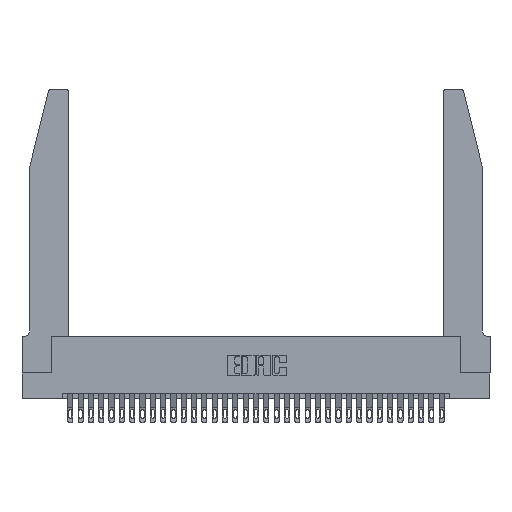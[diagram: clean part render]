
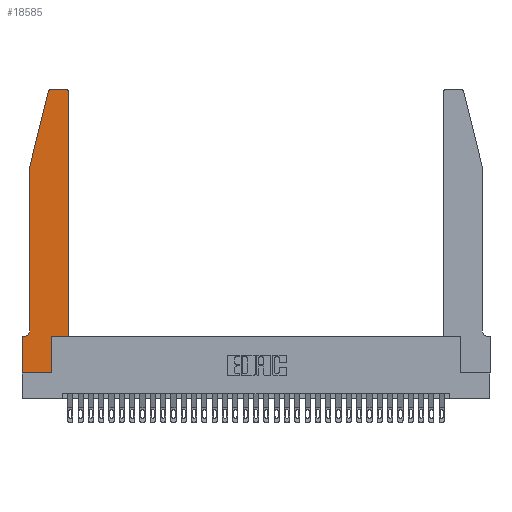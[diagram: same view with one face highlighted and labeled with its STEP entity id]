
A CAD part, top view. The second image highlights one B-rep face of the part: STEP entity #18585.
In plain terms, the highlighted planar face has unit normal (0, 0, 1).
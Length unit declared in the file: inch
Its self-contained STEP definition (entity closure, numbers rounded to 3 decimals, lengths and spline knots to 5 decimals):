
#20 = EDGE_LOOP ( 'NONE', ( #24383, #28133, #33479, #28263, #9314, #33963, #3796, #21470, #34028, #24798, #11192, #2394 ) ) ;
#1036 = DIRECTION ( 'NONE',  ( 0., 1., 0. ) ) ;
#1741 = DIRECTION ( 'NONE',  ( 1., 0., 0. ) ) ;
#1934 = AXIS2_PLACEMENT_3D ( 'NONE', #31830, #33931, #18137 ) ;
#2394 = ORIENTED_EDGE ( 'NONE', *, *, #11421, .T. ) ;
#2669 = VECTOR ( 'NONE', #12500, 39.37008 ) ;
#3556 = EDGE_CURVE ( 'NONE', #12029, #30314, #17041, .T. ) ;
#3796 = ORIENTED_EDGE ( 'NONE', *, *, #12665, .T. ) ;
#3810 = LINE ( 'NONE', #32622, #26103 ) ;
#4499 = LINE ( 'NONE', #11908, #25490 ) ;
#4633 = LINE ( 'NONE', #25714, #8369 ) ;
#5110 = VERTEX_POINT ( 'NONE', #10201 ) ;
#5418 = VERTEX_POINT ( 'NONE', #31529 ) ;
#5482 = VERTEX_POINT ( 'NONE', #34102 ) ;
#5614 = EDGE_CURVE ( 'NONE', #20207, #5418, #29988, .T. ) ;
#6049 = DIRECTION ( 'NONE',  ( 1., 0., 0. ) ) ;
#6321 = CARTESIAN_POINT ( 'NONE',  ( 0.4505, 2.72, 0.37 ) ) ;
#6489 = EDGE_CURVE ( 'NONE', #10993, #6961, #17718, .T. ) ;
#6961 = VERTEX_POINT ( 'NONE', #12233 ) ;
#7520 = VECTOR ( 'NONE', #23415, 39.37008 ) ;
#8369 = VECTOR ( 'NONE', #31286, 39.37008 ) ;
#8616 = CARTESIAN_POINT ( 'NONE',  ( 0., 0.35, 0.37 ) ) ;
#9282 = EDGE_CURVE ( 'NONE', #5418, #12029, #10143, .T. ) ;
#9314 = ORIENTED_EDGE ( 'NONE', *, *, #3556, .T. ) ;
#9832 = EDGE_CURVE ( 'NONE', #5110, #13591, #3810, .T. ) ;
#10000 = VERTEX_POINT ( 'NONE', #6321 ) ;
#10143 = LINE ( 'NONE', #28679, #30764 ) ;
#10201 = CARTESIAN_POINT ( 'NONE',  ( 0.4205, 2.75, 0.37 ) ) ;
#10918 = CARTESIAN_POINT ( 'NONE',  ( 0.25487, 2.72718, 0.37 ) ) ;
#10931 = EDGE_CURVE ( 'NONE', #27137, #5482, #4633, .T. ) ;
#10993 = VERTEX_POINT ( 'NONE', #21674 ) ;
#11192 = ORIENTED_EDGE ( 'NONE', *, *, #14235, .T. ) ;
#11421 = EDGE_CURVE ( 'NONE', #10000, #5110, #16294, .T. ) ;
#11894 = AXIS2_PLACEMENT_3D ( 'NONE', #8616, #19373, #6049 ) ;
#11908 = CARTESIAN_POINT ( 'NONE',  ( 0., 0., 0.37 ) ) ;
#12029 = VERTEX_POINT ( 'NONE', #34087 ) ;
#12233 = CARTESIAN_POINT ( 'NONE',  ( 0.4505, 0.35, 0.37 ) ) ;
#12500 = DIRECTION ( 'NONE',  ( -0.239, -0.971, 0. ) ) ;
#12665 = EDGE_CURVE ( 'NONE', #13957, #27137, #4499, .T. ) ;
#12746 = CIRCLE ( 'NONE', #1934, 0.03 ) ;
#13058 = CARTESIAN_POINT ( 'NONE',  ( 0., 0.35, 0.37 ) ) ;
#13591 = VERTEX_POINT ( 'NONE', #25561 ) ;
#13957 = VERTEX_POINT ( 'NONE', #13058 ) ;
#14192 = CARTESIAN_POINT ( 'NONE',  ( 0.4505, 0.35, 0.37 ) ) ;
#14235 = EDGE_CURVE ( 'NONE', #6961, #10000, #25348, .T. ) ;
#15864 = LINE ( 'NONE', #33928, #7520 ) ;
#16294 = CIRCLE ( 'NONE', #24153, 0.03 ) ;
#16435 = LINE ( 'NONE', #25525, #33722 ) ;
#17041 = CIRCLE ( 'NONE', #17306, 0.07 ) ;
#17306 = AXIS2_PLACEMENT_3D ( 'NONE', #25915, #20619, #22845 ) ;
#17718 = LINE ( 'NONE', #19577, #33281 ) ;
#18137 = DIRECTION ( 'NONE',  ( 1., 0., 0. ) ) ;
#18141 = EDGE_CURVE ( 'NONE', #30314, #13957, #16435, .T. ) ;
#18178 = DIRECTION ( 'NONE',  ( 0., 0., 1. ) ) ;
#18585 = ADVANCED_FACE ( 'NONE', ( #23561 ), #21867, .T. ) ;
#19373 = DIRECTION ( 'NONE',  ( 0., 0., 1. ) ) ;
#19577 = CARTESIAN_POINT ( 'NONE',  ( 0.4505, 0.35, 0.37 ) ) ;
#20207 = VERTEX_POINT ( 'NONE', #10918 ) ;
#20246 = DIRECTION ( 'NONE',  ( 0., -1., 0. ) ) ;
#20619 = DIRECTION ( 'NONE',  ( 0., 0., -1. ) ) ;
#20823 = CARTESIAN_POINT ( 'NONE',  ( 0.0755, 2., 0.37 ) ) ;
#21470 = ORIENTED_EDGE ( 'NONE', *, *, #10931, .T. ) ;
#21674 = CARTESIAN_POINT ( 'NONE',  ( 0.2865, 0.35, 0.37 ) ) ;
#21867 = PLANE ( 'NONE',  #11894 ) ;
#22329 = DIRECTION ( 'NONE',  ( -1., 0., 0. ) ) ;
#22604 = EDGE_CURVE ( 'NONE', #13591, #20207, #12746, .T. ) ;
#22845 = DIRECTION ( 'NONE',  ( -1., 0., 0. ) ) ;
#23415 = DIRECTION ( 'NONE',  ( 0., 1., 0. ) ) ;
#23561 = FACE_OUTER_BOUND ( 'NONE', #20, .T. ) ;
#24153 = AXIS2_PLACEMENT_3D ( 'NONE', #34327, #18178, #31867 ) ;
#24383 = ORIENTED_EDGE ( 'NONE', *, *, #9832, .T. ) ;
#24798 = ORIENTED_EDGE ( 'NONE', *, *, #6489, .T. ) ;
#25348 = LINE ( 'NONE', #14192, #32127 ) ;
#25490 = VECTOR ( 'NONE', #20246, 39.37008 ) ;
#25525 = CARTESIAN_POINT ( 'NONE',  ( 0.0755, 0.35, 0.37 ) ) ;
#25561 = CARTESIAN_POINT ( 'NONE',  ( 0.284, 2.75, 0.37 ) ) ;
#25714 = CARTESIAN_POINT ( 'NONE',  ( 0., 0., 0.37 ) ) ;
#25915 = CARTESIAN_POINT ( 'NONE',  ( 0.0055, 0.42, 0.37 ) ) ;
#26103 = VECTOR ( 'NONE', #22329, 39.37008 ) ;
#26412 = EDGE_CURVE ( 'NONE', #5482, #10993, #15864, .T. ) ;
#27137 = VERTEX_POINT ( 'NONE', #32244 ) ;
#28133 = ORIENTED_EDGE ( 'NONE', *, *, #22604, .T. ) ;
#28263 = ORIENTED_EDGE ( 'NONE', *, *, #9282, .T. ) ;
#28679 = CARTESIAN_POINT ( 'NONE',  ( 0.0755, 2., 0.37 ) ) ;
#29988 = LINE ( 'NONE', #20823, #2669 ) ;
#30314 = VERTEX_POINT ( 'NONE', #32644 ) ;
#30764 = VECTOR ( 'NONE', #34335, 39.37008 ) ;
#30844 = DIRECTION ( 'NONE',  ( -1., 0., 0. ) ) ;
#31286 = DIRECTION ( 'NONE',  ( 1., 0., 0. ) ) ;
#31529 = CARTESIAN_POINT ( 'NONE',  ( 0.0755, 2., 0.37 ) ) ;
#31830 = CARTESIAN_POINT ( 'NONE',  ( 0.284, 2.72, 0.37 ) ) ;
#31867 = DIRECTION ( 'NONE',  ( 1., 0., 0. ) ) ;
#32127 = VECTOR ( 'NONE', #1036, 39.37008 ) ;
#32244 = CARTESIAN_POINT ( 'NONE',  ( 0., 0., 0.37 ) ) ;
#32622 = CARTESIAN_POINT ( 'NONE',  ( 0.2605, 2.75, 0.37 ) ) ;
#32644 = CARTESIAN_POINT ( 'NONE',  ( 0.0055, 0.35, 0.37 ) ) ;
#33281 = VECTOR ( 'NONE', #1741, 39.37008 ) ;
#33479 = ORIENTED_EDGE ( 'NONE', *, *, #5614, .T. ) ;
#33722 = VECTOR ( 'NONE', #30844, 39.37008 ) ;
#33928 = CARTESIAN_POINT ( 'NONE',  ( 0.2865, 0.35, 0.37 ) ) ;
#33931 = DIRECTION ( 'NONE',  ( 0., 0., 1. ) ) ;
#33963 = ORIENTED_EDGE ( 'NONE', *, *, #18141, .T. ) ;
#34028 = ORIENTED_EDGE ( 'NONE', *, *, #26412, .T. ) ;
#34087 = CARTESIAN_POINT ( 'NONE',  ( 0.0755, 0.42, 0.37 ) ) ;
#34102 = CARTESIAN_POINT ( 'NONE',  ( 0.2865, 0., 0.37 ) ) ;
#34327 = CARTESIAN_POINT ( 'NONE',  ( 0.4205, 2.72, 0.37 ) ) ;
#34335 = DIRECTION ( 'NONE',  ( 0., -1., 0. ) ) ;
